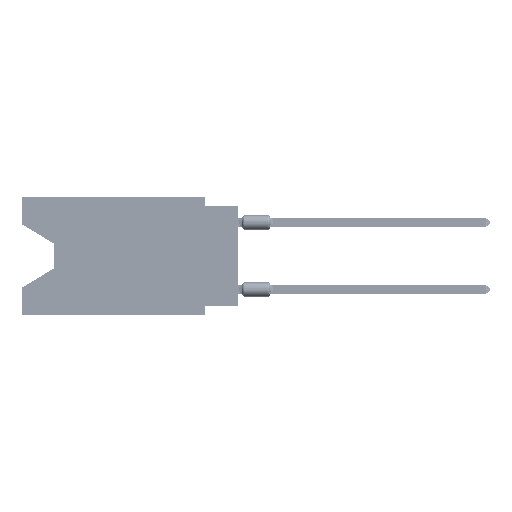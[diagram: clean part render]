
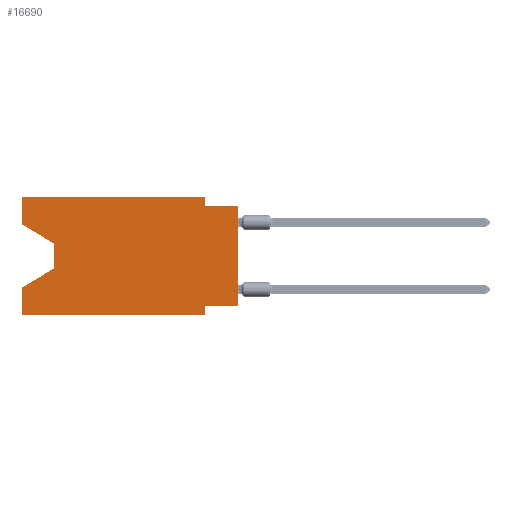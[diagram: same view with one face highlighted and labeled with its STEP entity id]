
A CAD part, left-side view. The second image highlights one B-rep face of the part: STEP entity #16690.
In plain terms, the highlighted planar face has unit normal (-1, 0, 0).
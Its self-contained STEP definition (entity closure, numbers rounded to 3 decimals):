
#583 = ORIENTED_EDGE ( 'NONE', *, *, #34183, .T. ) ;
#1144 = VERTEX_POINT ( 'NONE', #44941 ) ;
#1646 = ORIENTED_EDGE ( 'NONE', *, *, #67050, .F. ) ;
#2124 = DIRECTION ( 'NONE',  ( 0., -0.855, -0.519 ) ) ;
#2228 = VERTEX_POINT ( 'NONE', #25529 ) ;
#2482 = VERTEX_POINT ( 'NONE', #2945 ) ;
#2918 = VECTOR ( 'NONE', #22147, 1000. ) ;
#2945 = CARTESIAN_POINT ( 'NONE',  ( 0., 2.54, -8.255 ) ) ;
#3516 = CARTESIAN_POINT ( 'NONE',  ( 0., 2.54, 0. ) ) ;
#4922 = CARTESIAN_POINT ( 'NONE',  ( 0., 0., -8.255 ) ) ;
#5321 = DIRECTION ( 'NONE',  ( 0., 0., -1. ) ) ;
#7088 = CARTESIAN_POINT ( 'NONE',  ( 0., 0., -8.255 ) ) ;
#7221 = CARTESIAN_POINT ( 'NONE',  ( 0., 13.97, -5.385 ) ) ;
#7415 = CARTESIAN_POINT ( 'NONE',  ( 0., 16.383, 0. ) ) ;
#8436 = ORIENTED_EDGE ( 'NONE', *, *, #65926, .T. ) ;
#8913 = EDGE_CURVE ( 'NONE', #57232, #58489, #72403, .T. ) ;
#10574 = CARTESIAN_POINT ( 'NONE',  ( 0., 13.97, -3.505 ) ) ;
#11513 = PLANE ( 'NONE',  #66005 ) ;
#12156 = CARTESIAN_POINT ( 'NONE',  ( 0., 2.54, -0.635 ) ) ;
#13001 = VERTEX_POINT ( 'NONE', #12156 ) ;
#13259 = EDGE_CURVE ( 'NONE', #48063, #2482, #60414, .T. ) ;
#14267 = LINE ( 'NONE', #25948, #38532 ) ;
#14404 = CARTESIAN_POINT ( 'NONE',  ( 0., 16.383, 0. ) ) ;
#15000 = LINE ( 'NONE', #37982, #58140 ) ;
#16030 = LINE ( 'NONE', #10574, #39555 ) ;
#16690 = ADVANCED_FACE ( 'NONE', ( #70675 ), #11513, .F. ) ;
#17620 = LINE ( 'NONE', #59648, #68857 ) ;
#18613 = VECTOR ( 'NONE', #54572, 1000. ) ;
#19628 = CARTESIAN_POINT ( 'NONE',  ( 0., 16.383, -2.038 ) ) ;
#19893 = ORIENTED_EDGE ( 'NONE', *, *, #76406, .F. ) ;
#22147 = DIRECTION ( 'NONE',  ( 0., -1., 0. ) ) ;
#25529 = CARTESIAN_POINT ( 'NONE',  ( 0., 2.54, -8.89 ) ) ;
#25660 = ORIENTED_EDGE ( 'NONE', *, *, #13259, .F. ) ;
#25948 = CARTESIAN_POINT ( 'NONE',  ( 0., 16.383, 0. ) ) ;
#26428 = DIRECTION ( 'NONE',  ( 0., -1., 0. ) ) ;
#27993 = LINE ( 'NONE', #63420, #2918 ) ;
#28056 = DIRECTION ( 'NONE',  ( 0., 0., 1. ) ) ;
#28379 = VECTOR ( 'NONE', #28056, 1000. ) ;
#29161 = ORIENTED_EDGE ( 'NONE', *, *, #69939, .F. ) ;
#33483 = LINE ( 'NONE', #3516, #67907 ) ;
#34183 = EDGE_CURVE ( 'NONE', #48063, #58405, #64244, .T. ) ;
#37982 = CARTESIAN_POINT ( 'NONE',  ( 0., 2.54, -8.89 ) ) ;
#38532 = VECTOR ( 'NONE', #43836, 1000. ) ;
#38778 = ORIENTED_EDGE ( 'NONE', *, *, #55677, .F. ) ;
#39555 = VECTOR ( 'NONE', #51060, 1000. ) ;
#40452 = CARTESIAN_POINT ( 'NONE',  ( 0., 13.97, -5.385 ) ) ;
#40668 = VERTEX_POINT ( 'NONE', #65574 ) ;
#42828 = VERTEX_POINT ( 'NONE', #14404 ) ;
#43272 = VECTOR ( 'NONE', #2124, 1000. ) ;
#43300 = VECTOR ( 'NONE', #64583, 1000. ) ;
#43836 = DIRECTION ( 'NONE',  ( 0., -1., 0. ) ) ;
#44941 = CARTESIAN_POINT ( 'NONE',  ( 0., 2.54, 0. ) ) ;
#45568 = CARTESIAN_POINT ( 'NONE',  ( 0., 0., 0. ) ) ;
#47692 = DIRECTION ( 'NONE',  ( 1., 0., 0. ) ) ;
#48063 = VERTEX_POINT ( 'NONE', #4922 ) ;
#48234 = CARTESIAN_POINT ( 'NONE',  ( 0., 0., -0.635 ) ) ;
#48329 = VERTEX_POINT ( 'NONE', #7221 ) ;
#49378 = CARTESIAN_POINT ( 'NONE',  ( 0., 16.383, -8.89 ) ) ;
#49787 = CARTESIAN_POINT ( 'NONE',  ( 0., 16.383, -6.852 ) ) ;
#51060 = DIRECTION ( 'NONE',  ( 0., 0., -1. ) ) ;
#51862 = EDGE_LOOP ( 'NONE', ( #62807, #8436, #58761, #62443, #67012, #1646, #25660, #583, #58210, #38778, #29161, #19893 ) ) ;
#52246 = VERTEX_POINT ( 'NONE', #53478 ) ;
#52272 = DIRECTION ( 'NONE',  ( 0., 0., 1. ) ) ;
#53478 = CARTESIAN_POINT ( 'NONE',  ( 0., 13.97, -3.505 ) ) ;
#54505 = DIRECTION ( 'NONE',  ( 0., 0., 1. ) ) ;
#54532 = VECTOR ( 'NONE', #54505, 1000. ) ;
#54572 = DIRECTION ( 'NONE',  ( 0., 1., 0. ) ) ;
#55677 = EDGE_CURVE ( 'NONE', #1144, #13001, #33483, .T. ) ;
#57168 = EDGE_CURVE ( 'NONE', #13001, #58405, #68062, .T. ) ;
#57232 = VERTEX_POINT ( 'NONE', #49378 ) ;
#58037 = EDGE_CURVE ( 'NONE', #40668, #52246, #73339, .T. ) ;
#58140 = VECTOR ( 'NONE', #61337, 1000. ) ;
#58210 = ORIENTED_EDGE ( 'NONE', *, *, #57168, .F. ) ;
#58405 = VERTEX_POINT ( 'NONE', #48234 ) ;
#58489 = VERTEX_POINT ( 'NONE', #49787 ) ;
#58761 = ORIENTED_EDGE ( 'NONE', *, *, #67619, .T. ) ;
#59116 = LINE ( 'NONE', #40452, #43300 ) ;
#59648 = CARTESIAN_POINT ( 'NONE',  ( 0., 16.383, 0. ) ) ;
#60414 = LINE ( 'NONE', #7088, #18613 ) ;
#61337 = DIRECTION ( 'NONE',  ( 0., 0., -1. ) ) ;
#62443 = ORIENTED_EDGE ( 'NONE', *, *, #8913, .F. ) ;
#62807 = ORIENTED_EDGE ( 'NONE', *, *, #58037, .T. ) ;
#62981 = CARTESIAN_POINT ( 'NONE',  ( 0., 0., -0.635 ) ) ;
#63420 = CARTESIAN_POINT ( 'NONE',  ( 0., 16.383, -8.89 ) ) ;
#64244 = LINE ( 'NONE', #45568, #28379 ) ;
#64583 = DIRECTION ( 'NONE',  ( 0., 0.855, -0.519 ) ) ;
#65574 = CARTESIAN_POINT ( 'NONE',  ( 0., 16.383, -2.038 ) ) ;
#65926 = EDGE_CURVE ( 'NONE', #52246, #48329, #16030, .T. ) ;
#65988 = CARTESIAN_POINT ( 'NONE',  ( 0., 16.383, 0. ) ) ;
#66005 = AXIS2_PLACEMENT_3D ( 'NONE', #65988, #47692, #76881 ) ;
#67012 = ORIENTED_EDGE ( 'NONE', *, *, #75111, .T. ) ;
#67050 = EDGE_CURVE ( 'NONE', #2482, #2228, #15000, .T. ) ;
#67619 = EDGE_CURVE ( 'NONE', #48329, #58489, #59116, .T. ) ;
#67907 = VECTOR ( 'NONE', #5321, 1000. ) ;
#68062 = LINE ( 'NONE', #62981, #70496 ) ;
#68857 = VECTOR ( 'NONE', #52272, 1000. ) ;
#69939 = EDGE_CURVE ( 'NONE', #42828, #1144, #14267, .T. ) ;
#70496 = VECTOR ( 'NONE', #26428, 1000. ) ;
#70675 = FACE_OUTER_BOUND ( 'NONE', #51862, .T. ) ;
#72403 = LINE ( 'NONE', #7415, #54532 ) ;
#73339 = LINE ( 'NONE', #19628, #43272 ) ;
#75111 = EDGE_CURVE ( 'NONE', #57232, #2228, #27993, .T. ) ;
#76406 = EDGE_CURVE ( 'NONE', #40668, #42828, #17620, .T. ) ;
#76881 = DIRECTION ( 'NONE',  ( 0., 0., -1. ) ) ;
